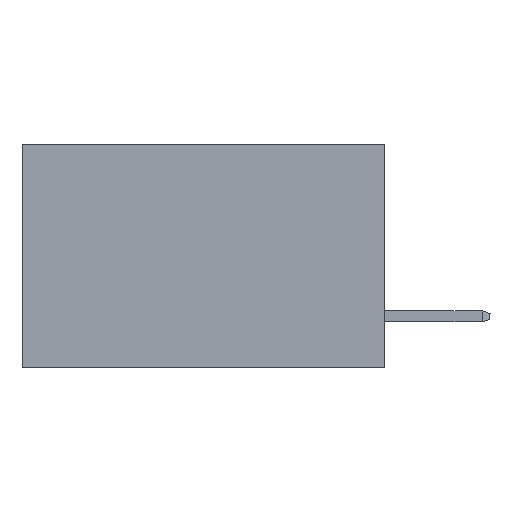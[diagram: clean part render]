
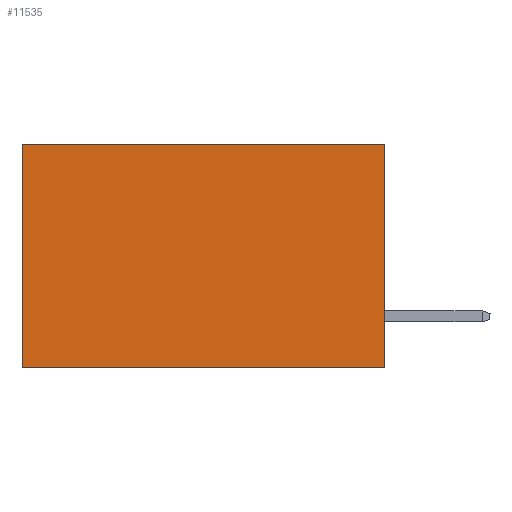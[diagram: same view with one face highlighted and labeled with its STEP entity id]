
A CAD part, left-side view. The second image highlights one B-rep face of the part: STEP entity #11535.
In plain terms, the highlighted planar face has unit normal (-1, 0, 0).
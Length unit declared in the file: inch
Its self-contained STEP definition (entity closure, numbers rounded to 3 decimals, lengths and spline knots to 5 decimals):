
#24 = CARTESIAN_POINT ( 'NONE',  ( 0.2615, 0., 0. ) ) ;
#107 = LINE ( 'NONE', #3830, #11983 ) ;
#203 = VERTEX_POINT ( 'NONE', #4406 ) ;
#934 = ORIENTED_EDGE ( 'NONE', *, *, #2488, .F. ) ;
#1487 = CARTESIAN_POINT ( 'NONE',  ( 0.2615, 0., -0.37 ) ) ;
#1798 = CARTESIAN_POINT ( 'NONE',  ( 0.2615, 0., -0.37 ) ) ;
#1905 = VECTOR ( 'NONE', #9312, 39.37008 ) ;
#1954 = DIRECTION ( 'NONE',  ( 0., 0., -1. ) ) ;
#2005 = DIRECTION ( 'NONE',  ( 0., 0., -1. ) ) ;
#2464 = VECTOR ( 'NONE', #11544, 39.37008 ) ;
#2488 = EDGE_CURVE ( 'NONE', #6738, #5535, #10047, .T. ) ;
#3830 = CARTESIAN_POINT ( 'NONE',  ( 0.2615, 0.6, -0.37 ) ) ;
#3975 = ORIENTED_EDGE ( 'NONE', *, *, #6473, .T. ) ;
#4115 = CARTESIAN_POINT ( 'NONE',  ( 0.2615, 0., -0.37 ) ) ;
#4406 = CARTESIAN_POINT ( 'NONE',  ( 0.2615, 0.6, 0. ) ) ;
#4585 = PLANE ( 'NONE',  #10784 ) ;
#4768 = FACE_OUTER_BOUND ( 'NONE', #6391, .T. ) ;
#5198 = CARTESIAN_POINT ( 'NONE',  ( 0.2615, 0.6, -0.37 ) ) ;
#5469 = LINE ( 'NONE', #24, #9097 ) ;
#5535 = VERTEX_POINT ( 'NONE', #5198 ) ;
#5749 = CARTESIAN_POINT ( 'NONE',  ( 0.2615, 0., -0.37 ) ) ;
#5815 = VERTEX_POINT ( 'NONE', #7829 ) ;
#6391 = EDGE_LOOP ( 'NONE', ( #10353, #934, #6496, #3975 ) ) ;
#6473 = EDGE_CURVE ( 'NONE', #5815, #203, #5469, .T. ) ;
#6496 = ORIENTED_EDGE ( 'NONE', *, *, #9581, .F. ) ;
#6738 = VERTEX_POINT ( 'NONE', #1487 ) ;
#7829 = CARTESIAN_POINT ( 'NONE',  ( 0.2615, 0., 0. ) ) ;
#8541 = EDGE_CURVE ( 'NONE', #203, #5535, #107, .T. ) ;
#9097 = VECTOR ( 'NONE', #10998, 39.37008 ) ;
#9312 = DIRECTION ( 'NONE',  ( 0., 1., 0. ) ) ;
#9400 = DIRECTION ( 'NONE',  ( 1., 0., 0. ) ) ;
#9581 = EDGE_CURVE ( 'NONE', #5815, #6738, #10467, .T. ) ;
#10047 = LINE ( 'NONE', #1798, #1905 ) ;
#10353 = ORIENTED_EDGE ( 'NONE', *, *, #8541, .T. ) ;
#10467 = LINE ( 'NONE', #4115, #2464 ) ;
#10784 = AXIS2_PLACEMENT_3D ( 'NONE', #5749, #9400, #1954 ) ;
#10998 = DIRECTION ( 'NONE',  ( 0., 1., 0. ) ) ;
#11535 = ADVANCED_FACE ( 'NONE', ( #4768 ), #4585, .F. ) ;
#11544 = DIRECTION ( 'NONE',  ( 0., 0., -1. ) ) ;
#11983 = VECTOR ( 'NONE', #2005, 39.37008 ) ;
